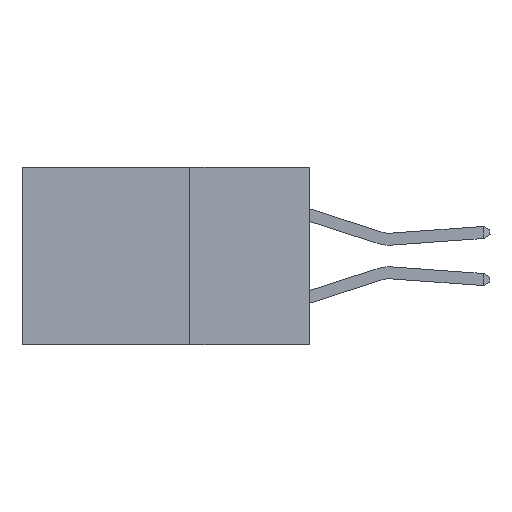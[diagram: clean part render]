
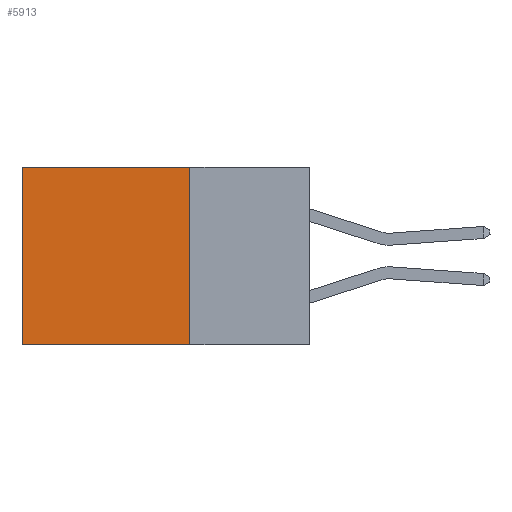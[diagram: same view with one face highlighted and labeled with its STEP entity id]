
A CAD part, left-side view. The second image highlights one B-rep face of the part: STEP entity #5913.
In plain terms, the highlighted planar face has unit normal (-1, 0, 0).
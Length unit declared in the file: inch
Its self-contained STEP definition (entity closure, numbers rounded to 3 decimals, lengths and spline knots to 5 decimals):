
#1302 = LINE ( 'NONE', #5727, #14480 ) ;
#1831 = VECTOR ( 'NONE', #13020, 39.37008 ) ;
#1908 = CARTESIAN_POINT ( 'NONE',  ( 0.298, 0.6, 0. ) ) ;
#3634 = PLANE ( 'NONE',  #11587 ) ;
#4255 = VERTEX_POINT ( 'NONE', #18220 ) ;
#4927 = VERTEX_POINT ( 'NONE', #6030 ) ;
#5486 = LINE ( 'NONE', #12349, #17407 ) ;
#5727 = CARTESIAN_POINT ( 'NONE',  ( 0.298, 0.25, -0.37 ) ) ;
#5913 = ADVANCED_FACE ( 'NONE', ( #14073 ), #3634, .F. ) ;
#6030 = CARTESIAN_POINT ( 'NONE',  ( 0.298, 0.25, -0.37 ) ) ;
#6430 = VERTEX_POINT ( 'NONE', #6477 ) ;
#6477 = CARTESIAN_POINT ( 'NONE',  ( 0.298, 0.6, 0. ) ) ;
#7047 = VERTEX_POINT ( 'NONE', #15516 ) ;
#7768 = CARTESIAN_POINT ( 'NONE',  ( 0.298, 0.25, 0. ) ) ;
#7776 = CARTESIAN_POINT ( 'NONE',  ( 0.298, 0.25, 0. ) ) ;
#7798 = DIRECTION ( 'NONE',  ( 0., 0., -1. ) ) ;
#7888 = DIRECTION ( 'NONE',  ( 1., 0., 0. ) ) ;
#9335 = DIRECTION ( 'NONE',  ( 0., 1., 0. ) ) ;
#9634 = ORIENTED_EDGE ( 'NONE', *, *, #14650, .T. ) ;
#9984 = ORIENTED_EDGE ( 'NONE', *, *, #19270, .F. ) ;
#10307 = VECTOR ( 'NONE', #9335, 39.37008 ) ;
#10432 = DIRECTION ( 'NONE',  ( 0., 1., 0. ) ) ;
#11587 = AXIS2_PLACEMENT_3D ( 'NONE', #7776, #7888, #7798 ) ;
#12349 = CARTESIAN_POINT ( 'NONE',  ( 0.298, 0.25, 0. ) ) ;
#12723 = EDGE_CURVE ( 'NONE', #7047, #4927, #5486, .T. ) ;
#13020 = DIRECTION ( 'NONE',  ( 0., 0., -1. ) ) ;
#14073 = FACE_OUTER_BOUND ( 'NONE', #16498, .T. ) ;
#14223 = EDGE_CURVE ( 'NONE', #6430, #4255, #14485, .T. ) ;
#14480 = VECTOR ( 'NONE', #10432, 39.37008 ) ;
#14485 = LINE ( 'NONE', #1908, #1831 ) ;
#14650 = EDGE_CURVE ( 'NONE', #7047, #6430, #18525, .T. ) ;
#15516 = CARTESIAN_POINT ( 'NONE',  ( 0.298, 0.25, 0. ) ) ;
#15525 = ORIENTED_EDGE ( 'NONE', *, *, #12723, .F. ) ;
#16498 = EDGE_LOOP ( 'NONE', ( #17896, #9984, #15525, #9634 ) ) ;
#17407 = VECTOR ( 'NONE', #19974, 39.37008 ) ;
#17896 = ORIENTED_EDGE ( 'NONE', *, *, #14223, .T. ) ;
#18220 = CARTESIAN_POINT ( 'NONE',  ( 0.298, 0.6, -0.37 ) ) ;
#18525 = LINE ( 'NONE', #7768, #10307 ) ;
#19270 = EDGE_CURVE ( 'NONE', #4927, #4255, #1302, .T. ) ;
#19974 = DIRECTION ( 'NONE',  ( 0., 0., -1. ) ) ;
